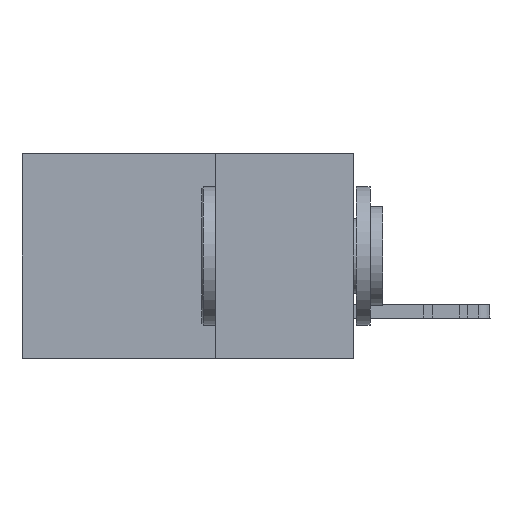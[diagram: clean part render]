
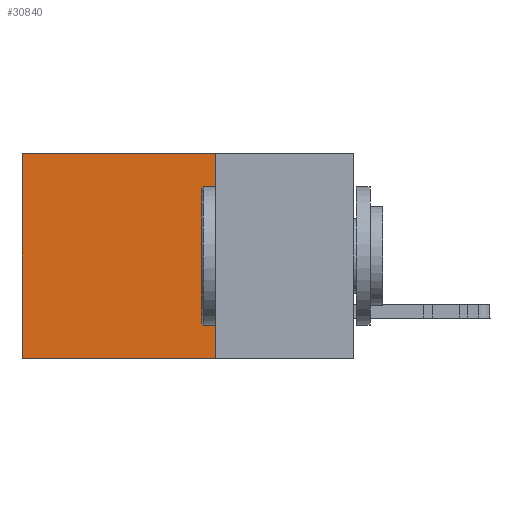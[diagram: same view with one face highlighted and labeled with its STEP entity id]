
A CAD part, left-side view. The second image highlights one B-rep face of the part: STEP entity #30840.
In plain terms, the highlighted planar face has unit normal (-1, 0, 0).
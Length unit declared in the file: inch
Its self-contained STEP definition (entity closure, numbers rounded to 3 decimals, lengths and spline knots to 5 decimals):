
#1524 = ORIENTED_EDGE ( 'NONE', *, *, #40452, .F. ) ;
#1923 = VERTEX_POINT ( 'NONE', #20521 ) ;
#3581 = EDGE_CURVE ( 'NONE', #32027, #1923, #27297, .T. ) ;
#4302 = EDGE_CURVE ( 'NONE', #36339, #7805, #7181, .T. ) ;
#6233 = DIRECTION ( 'NONE',  ( 0., 0., -1. ) ) ;
#6690 = DIRECTION ( 'NONE',  ( 0., 1., 0. ) ) ;
#7181 = LINE ( 'NONE', #7391, #29435 ) ;
#7391 = CARTESIAN_POINT ( 'NONE',  ( 0.2875, 0.25, -0.37 ) ) ;
#7805 = VERTEX_POINT ( 'NONE', #32377 ) ;
#8342 = VECTOR ( 'NONE', #6233, 39.37008 ) ;
#8498 = ORIENTED_EDGE ( 'NONE', *, *, #3581, .T. ) ;
#8828 = AXIS2_PLACEMENT_3D ( 'NONE', #30033, #39661, #13580 ) ;
#8834 = LINE ( 'NONE', #19351, #32557 ) ;
#10470 = DIRECTION ( 'NONE',  ( 0., 1., 0. ) ) ;
#13140 = FACE_OUTER_BOUND ( 'NONE', #27811, .T. ) ;
#13580 = DIRECTION ( 'NONE',  ( 0., 0., -1. ) ) ;
#17071 = VECTOR ( 'NONE', #6690, 39.37008 ) ;
#18256 = CARTESIAN_POINT ( 'NONE',  ( 0.2875, 0.25, 0. ) ) ;
#18383 = ORIENTED_EDGE ( 'NONE', *, *, #32763, .T. ) ;
#19351 = CARTESIAN_POINT ( 'NONE',  ( 0.2875, 0.6, 0. ) ) ;
#19626 = CARTESIAN_POINT ( 'NONE',  ( 0.2875, 0.25, -0.37 ) ) ;
#20521 = CARTESIAN_POINT ( 'NONE',  ( 0.2875, 0.6, 0. ) ) ;
#21985 = DIRECTION ( 'NONE',  ( 0., 0., -1. ) ) ;
#26385 = ORIENTED_EDGE ( 'NONE', *, *, #4302, .F. ) ;
#27297 = LINE ( 'NONE', #40859, #17071 ) ;
#27811 = EDGE_LOOP ( 'NONE', ( #18383, #26385, #1524, #8498 ) ) ;
#29435 = VECTOR ( 'NONE', #10470, 39.37008 ) ;
#30033 = CARTESIAN_POINT ( 'NONE',  ( 0.2875, 0.25, 0. ) ) ;
#30252 = PLANE ( 'NONE',  #8828 ) ;
#30840 = ADVANCED_FACE ( 'NONE', ( #13140 ), #30252, .F. ) ;
#32027 = VERTEX_POINT ( 'NONE', #18256 ) ;
#32377 = CARTESIAN_POINT ( 'NONE',  ( 0.2875, 0.6, -0.37 ) ) ;
#32557 = VECTOR ( 'NONE', #21985, 39.37008 ) ;
#32763 = EDGE_CURVE ( 'NONE', #1923, #7805, #8834, .T. ) ;
#36273 = CARTESIAN_POINT ( 'NONE',  ( 0.2875, 0.25, 0. ) ) ;
#36339 = VERTEX_POINT ( 'NONE', #19626 ) ;
#39545 = LINE ( 'NONE', #36273, #8342 ) ;
#39661 = DIRECTION ( 'NONE',  ( 1., 0., 0. ) ) ;
#40452 = EDGE_CURVE ( 'NONE', #32027, #36339, #39545, .T. ) ;
#40859 = CARTESIAN_POINT ( 'NONE',  ( 0.2875, 0.25, 0. ) ) ;
